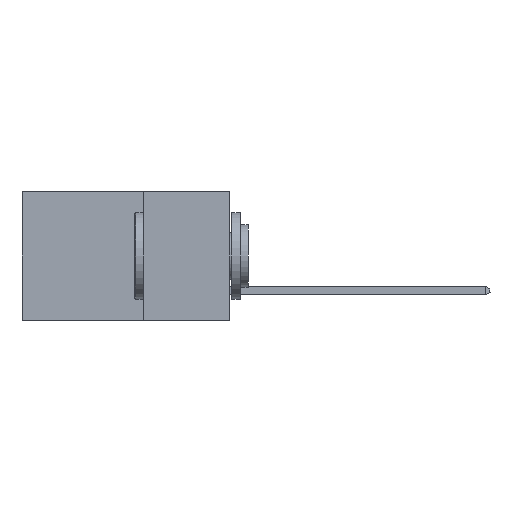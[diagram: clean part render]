
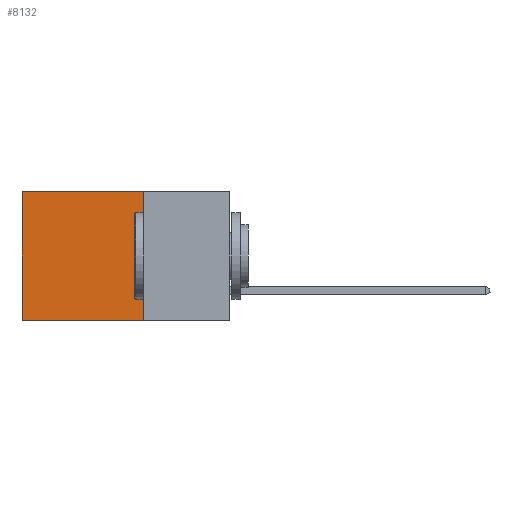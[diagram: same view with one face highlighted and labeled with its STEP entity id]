
A CAD part, left-side view. The second image highlights one B-rep face of the part: STEP entity #8132.
In plain terms, the highlighted planar face has unit normal (-1, 0, 0).
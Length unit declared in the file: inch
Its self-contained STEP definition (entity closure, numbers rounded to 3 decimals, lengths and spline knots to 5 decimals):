
#353 = VERTEX_POINT ( 'NONE', #14134 ) ;
#1734 = CARTESIAN_POINT ( 'NONE',  ( 0.298, 0.25, 0. ) ) ;
#1778 = EDGE_CURVE ( 'NONE', #4376, #26686, #6183, .T. ) ;
#1996 = VECTOR ( 'NONE', #27124, 39.37008 ) ;
#3116 = LINE ( 'NONE', #5408, #1996 ) ;
#3515 = CARTESIAN_POINT ( 'NONE',  ( 0.298, 0.25, 0. ) ) ;
#3828 = CARTESIAN_POINT ( 'NONE',  ( 0.298, 0.25, -0.37 ) ) ;
#4376 = VERTEX_POINT ( 'NONE', #18509 ) ;
#4759 = FACE_OUTER_BOUND ( 'NONE', #9404, .T. ) ;
#5408 = CARTESIAN_POINT ( 'NONE',  ( 0.298, 0.25, -0.37 ) ) ;
#6183 = LINE ( 'NONE', #9019, #17102 ) ;
#8132 = ADVANCED_FACE ( 'NONE', ( #4759 ), #30232, .F. ) ;
#8816 = DIRECTION ( 'NONE',  ( 0., 0., -1. ) ) ;
#9019 = CARTESIAN_POINT ( 'NONE',  ( 0.298, 0.25, 0. ) ) ;
#9338 = ORIENTED_EDGE ( 'NONE', *, *, #21589, .F. ) ;
#9404 = EDGE_LOOP ( 'NONE', ( #19771, #9338, #17739, #26489 ) ) ;
#10114 = LINE ( 'NONE', #15987, #28605 ) ;
#13387 = EDGE_CURVE ( 'NONE', #4376, #353, #26793, .T. ) ;
#14134 = CARTESIAN_POINT ( 'NONE',  ( 0.298, 0.6, 0. ) ) ;
#14290 = EDGE_CURVE ( 'NONE', #353, #22485, #10114, .T. ) ;
#15564 = DIRECTION ( 'NONE',  ( 1., 0., 0. ) ) ;
#15987 = CARTESIAN_POINT ( 'NONE',  ( 0.298, 0.6, 0. ) ) ;
#17102 = VECTOR ( 'NONE', #30759, 39.37008 ) ;
#17739 = ORIENTED_EDGE ( 'NONE', *, *, #1778, .F. ) ;
#18509 = CARTESIAN_POINT ( 'NONE',  ( 0.298, 0.25, 0. ) ) ;
#18866 = DIRECTION ( 'NONE',  ( 0., 1., 0. ) ) ;
#19771 = ORIENTED_EDGE ( 'NONE', *, *, #14290, .T. ) ;
#21589 = EDGE_CURVE ( 'NONE', #26686, #22485, #3116, .T. ) ;
#22269 = VECTOR ( 'NONE', #18866, 39.37008 ) ;
#22485 = VERTEX_POINT ( 'NONE', #23528 ) ;
#23528 = CARTESIAN_POINT ( 'NONE',  ( 0.298, 0.6, -0.37 ) ) ;
#26489 = ORIENTED_EDGE ( 'NONE', *, *, #13387, .T. ) ;
#26686 = VERTEX_POINT ( 'NONE', #3828 ) ;
#26793 = LINE ( 'NONE', #1734, #22269 ) ;
#27124 = DIRECTION ( 'NONE',  ( 0., 1., 0. ) ) ;
#27702 = DIRECTION ( 'NONE',  ( 0., 0., -1. ) ) ;
#28605 = VECTOR ( 'NONE', #8816, 39.37008 ) ;
#28898 = AXIS2_PLACEMENT_3D ( 'NONE', #3515, #15564, #27702 ) ;
#30232 = PLANE ( 'NONE',  #28898 ) ;
#30759 = DIRECTION ( 'NONE',  ( 0., 0., -1. ) ) ;
